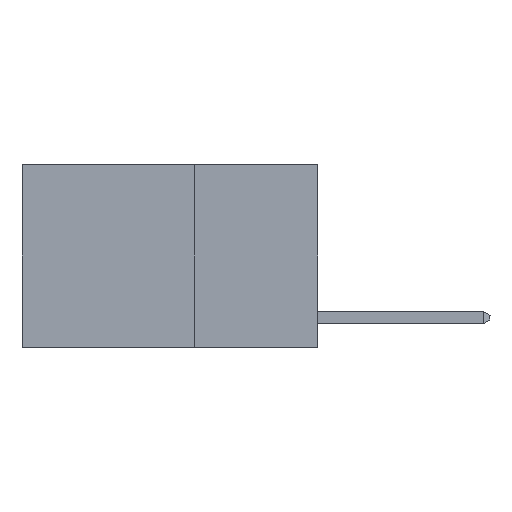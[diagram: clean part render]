
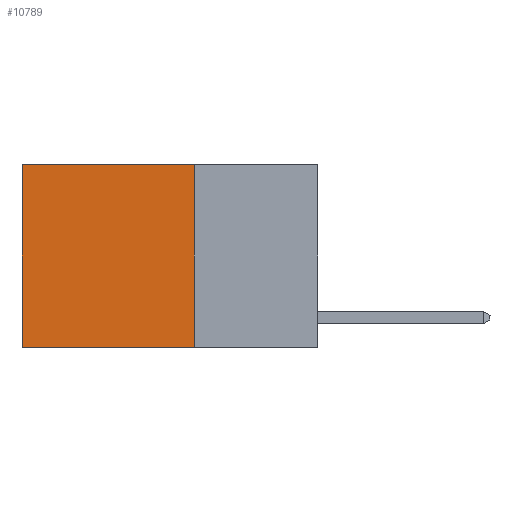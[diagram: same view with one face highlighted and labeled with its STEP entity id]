
A CAD part, left-side view. The second image highlights one B-rep face of the part: STEP entity #10789.
In plain terms, the highlighted planar face has unit normal (-1, 0, 0).
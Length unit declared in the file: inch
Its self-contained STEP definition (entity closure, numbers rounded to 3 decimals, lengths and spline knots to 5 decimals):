
#333 = AXIS2_PLACEMENT_3D ( 'NONE', #9882, #14475, #19167 ) ;
#1484 = DIRECTION ( 'NONE',  ( 0., 1., 0. ) ) ;
#1941 = EDGE_LOOP ( 'NONE', ( #11395, #4595, #8397, #11045 ) ) ;
#2181 = LINE ( 'NONE', #3475, #15148 ) ;
#2890 = EDGE_CURVE ( 'NONE', #4768, #5110, #19420, .T. ) ;
#3342 = LINE ( 'NONE', #7945, #8888 ) ;
#3475 = CARTESIAN_POINT ( 'NONE',  ( 0.2625, 0.25, -0.37 ) ) ;
#4029 = CARTESIAN_POINT ( 'NONE',  ( 0.2625, 0.6, 0. ) ) ;
#4161 = CARTESIAN_POINT ( 'NONE',  ( 0.2625, 0.6, 0. ) ) ;
#4595 = ORIENTED_EDGE ( 'NONE', *, *, #6133, .F. ) ;
#4768 = VERTEX_POINT ( 'NONE', #8377 ) ;
#4839 = DIRECTION ( 'NONE',  ( 0., 0., -1. ) ) ;
#5110 = VERTEX_POINT ( 'NONE', #4029 ) ;
#5774 = CARTESIAN_POINT ( 'NONE',  ( 0.2625, 0.25, 0. ) ) ;
#6009 = VERTEX_POINT ( 'NONE', #19342 ) ;
#6133 = EDGE_CURVE ( 'NONE', #11515, #6009, #2181, .T. ) ;
#7427 = EDGE_CURVE ( 'NONE', #4768, #11515, #3342, .T. ) ;
#7945 = CARTESIAN_POINT ( 'NONE',  ( 0.2625, 0.25, 0. ) ) ;
#8377 = CARTESIAN_POINT ( 'NONE',  ( 0.2625, 0.25, 0. ) ) ;
#8397 = ORIENTED_EDGE ( 'NONE', *, *, #7427, .F. ) ;
#8888 = VECTOR ( 'NONE', #4839, 39.37008 ) ;
#9477 = CARTESIAN_POINT ( 'NONE',  ( 0.2625, 0.25, -0.37 ) ) ;
#9882 = CARTESIAN_POINT ( 'NONE',  ( 0.2625, 0.25, 0. ) ) ;
#10789 = ADVANCED_FACE ( 'NONE', ( #17490 ), #16074, .F. ) ;
#11045 = ORIENTED_EDGE ( 'NONE', *, *, #2890, .T. ) ;
#11359 = DIRECTION ( 'NONE',  ( 0., 1., 0. ) ) ;
#11395 = ORIENTED_EDGE ( 'NONE', *, *, #17159, .T. ) ;
#11515 = VERTEX_POINT ( 'NONE', #9477 ) ;
#11827 = VECTOR ( 'NONE', #1484, 39.37008 ) ;
#11941 = LINE ( 'NONE', #4161, #17673 ) ;
#14475 = DIRECTION ( 'NONE',  ( 1., 0., 0. ) ) ;
#15148 = VECTOR ( 'NONE', #11359, 39.37008 ) ;
#16074 = PLANE ( 'NONE',  #333 ) ;
#17159 = EDGE_CURVE ( 'NONE', #5110, #6009, #11941, .T. ) ;
#17490 = FACE_OUTER_BOUND ( 'NONE', #1941, .T. ) ;
#17673 = VECTOR ( 'NONE', #17936, 39.37008 ) ;
#17936 = DIRECTION ( 'NONE',  ( 0., 0., -1. ) ) ;
#19167 = DIRECTION ( 'NONE',  ( 0., 0., -1. ) ) ;
#19342 = CARTESIAN_POINT ( 'NONE',  ( 0.2625, 0.6, -0.37 ) ) ;
#19420 = LINE ( 'NONE', #5774, #11827 ) ;
